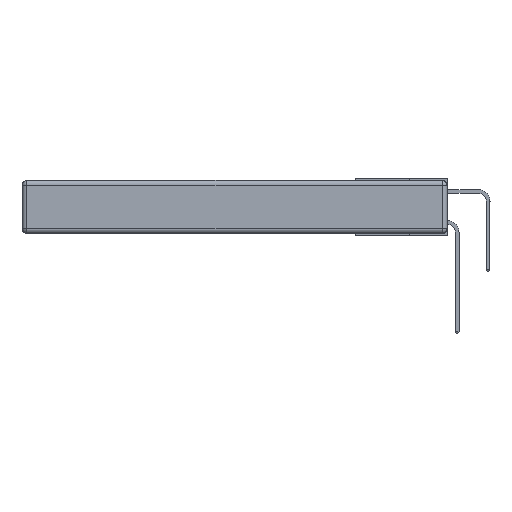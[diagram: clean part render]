
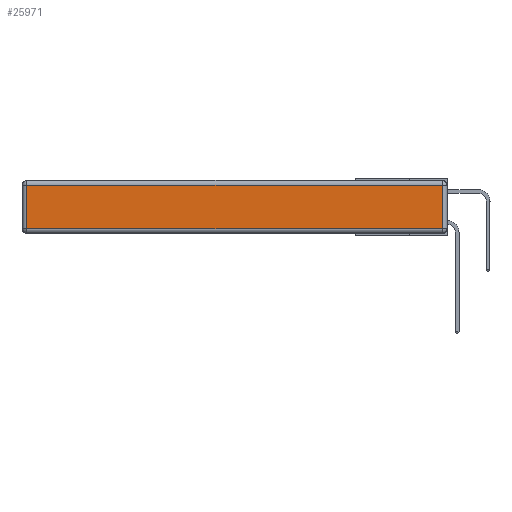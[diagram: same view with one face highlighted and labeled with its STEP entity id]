
A CAD part, left-side view. The second image highlights one B-rep face of the part: STEP entity #25971.
In plain terms, the highlighted planar face has unit normal (-1, 0, 0).
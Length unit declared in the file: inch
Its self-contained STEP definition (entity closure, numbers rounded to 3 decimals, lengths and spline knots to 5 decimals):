
#595 = ORIENTED_EDGE ( 'NONE', *, *, #8483, .T. ) ;
#3429 = CARTESIAN_POINT ( 'NONE',  ( 0., 2.75, -0.03 ) ) ;
#3767 = CARTESIAN_POINT ( 'NONE',  ( 0., 2.72, -0.03 ) ) ;
#4770 = ORIENTED_EDGE ( 'NONE', *, *, #29060, .T. ) ;
#5603 = PLANE ( 'NONE',  #21802 ) ;
#6480 = VECTOR ( 'NONE', #8121, 39.37008 ) ;
#7299 = DIRECTION ( 'NONE',  ( 0., 0., 1. ) ) ;
#8121 = DIRECTION ( 'NONE',  ( 0., -1., 0. ) ) ;
#8483 = EDGE_CURVE ( 'NONE', #13825, #28868, #11645, .T. ) ;
#9009 = DIRECTION ( 'NONE',  ( 0., 1., 0. ) ) ;
#9393 = VECTOR ( 'NONE', #7299, 39.37008 ) ;
#9468 = CARTESIAN_POINT ( 'NONE',  ( 0., 0.03, -0.03 ) ) ;
#11041 = CARTESIAN_POINT ( 'NONE',  ( 0., 0., -0.343 ) ) ;
#11645 = LINE ( 'NONE', #16534, #6480 ) ;
#11956 = EDGE_LOOP ( 'NONE', ( #595, #23325, #4770, #14337 ) ) ;
#13718 = VERTEX_POINT ( 'NONE', #9468 ) ;
#13825 = VERTEX_POINT ( 'NONE', #20857 ) ;
#13955 = CARTESIAN_POINT ( 'NONE',  ( 0., 0.03, -0.313 ) ) ;
#14167 = VERTEX_POINT ( 'NONE', #3767 ) ;
#14337 = ORIENTED_EDGE ( 'NONE', *, *, #20850, .T. ) ;
#16534 = CARTESIAN_POINT ( 'NONE',  ( 0., 0., -0.313 ) ) ;
#16701 = DIRECTION ( 'NONE',  ( 0., 0., 1. ) ) ;
#18091 = LINE ( 'NONE', #3429, #20692 ) ;
#20692 = VECTOR ( 'NONE', #9009, 39.37008 ) ;
#20850 = EDGE_CURVE ( 'NONE', #14167, #13825, #24719, .T. ) ;
#20857 = CARTESIAN_POINT ( 'NONE',  ( 0., 2.72, -0.313 ) ) ;
#21802 = AXIS2_PLACEMENT_3D ( 'NONE', #11041, #24960, #16701 ) ;
#22359 = DIRECTION ( 'NONE',  ( 0., 0., -1. ) ) ;
#23325 = ORIENTED_EDGE ( 'NONE', *, *, #26370, .T. ) ;
#23978 = CARTESIAN_POINT ( 'NONE',  ( 0., 0.03, -0.343 ) ) ;
#24125 = LINE ( 'NONE', #23978, #9393 ) ;
#24719 = LINE ( 'NONE', #28037, #28598 ) ;
#24960 = DIRECTION ( 'NONE',  ( -1., 0., 0. ) ) ;
#25971 = ADVANCED_FACE ( 'NONE', ( #35005 ), #5603, .T. ) ;
#26370 = EDGE_CURVE ( 'NONE', #28868, #13718, #24125, .T. ) ;
#28037 = CARTESIAN_POINT ( 'NONE',  ( 0., 2.72, -0.343 ) ) ;
#28598 = VECTOR ( 'NONE', #22359, 39.37008 ) ;
#28868 = VERTEX_POINT ( 'NONE', #13955 ) ;
#29060 = EDGE_CURVE ( 'NONE', #13718, #14167, #18091, .T. ) ;
#35005 = FACE_OUTER_BOUND ( 'NONE', #11956, .T. ) ;
